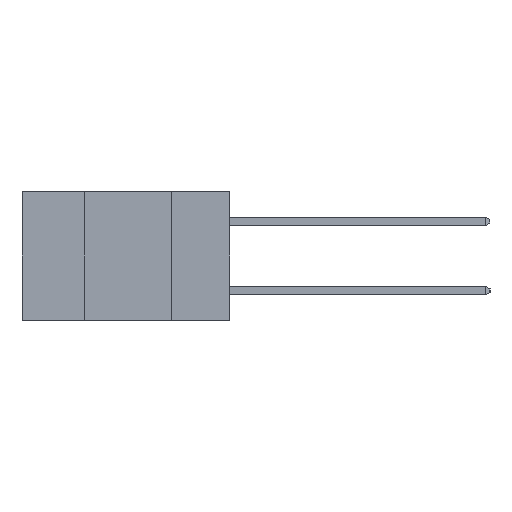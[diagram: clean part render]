
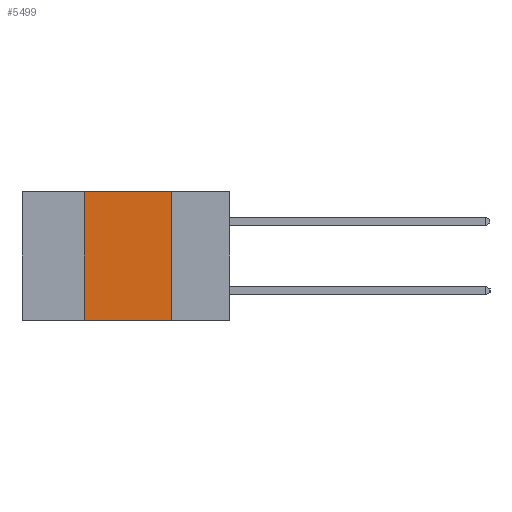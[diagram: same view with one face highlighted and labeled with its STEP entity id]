
A CAD part, left-side view. The second image highlights one B-rep face of the part: STEP entity #5499.
In plain terms, the highlighted planar face has unit normal (-1, 0, 0).
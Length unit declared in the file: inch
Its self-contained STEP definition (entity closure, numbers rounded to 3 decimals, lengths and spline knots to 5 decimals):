
#101 = VERTEX_POINT ( 'NONE', #11508 ) ;
#403 = DIRECTION ( 'NONE',  ( 0., 0., -1. ) ) ;
#486 = DIRECTION ( 'NONE',  ( 1., 0., 0. ) ) ;
#508 = PLANE ( 'NONE',  #15251 ) ;
#570 = CARTESIAN_POINT ( 'NONE',  ( 0., 0.6, 0. ) ) ;
#676 = VECTOR ( 'NONE', #7480, 39.37008 ) ;
#888 = FACE_OUTER_BOUND ( 'NONE', #13415, .T. ) ;
#1629 = VECTOR ( 'NONE', #9463, 39.37008 ) ;
#2603 = ORIENTED_EDGE ( 'NONE', *, *, #8192, .T. ) ;
#3342 = VERTEX_POINT ( 'NONE', #12175 ) ;
#4489 = ORIENTED_EDGE ( 'NONE', *, *, #6326, .F. ) ;
#4761 = LINE ( 'NONE', #9561, #1629 ) ;
#5140 = EDGE_CURVE ( 'NONE', #3342, #6577, #12088, .T. ) ;
#5459 = VECTOR ( 'NONE', #12535, 39.37008 ) ;
#5499 = ADVANCED_FACE ( 'NONE', ( #888 ), #508, .F. ) ;
#6326 = EDGE_CURVE ( 'NONE', #9936, #3342, #4761, .T. ) ;
#6577 = VERTEX_POINT ( 'NONE', #15065 ) ;
#6643 = EDGE_CURVE ( 'NONE', #6577, #101, #12986, .T. ) ;
#7480 = DIRECTION ( 'NONE',  ( 0., 0., -1. ) ) ;
#7483 = CARTESIAN_POINT ( 'NONE',  ( 0., 0.17, -0.37 ) ) ;
#7535 = LINE ( 'NONE', #12810, #5459 ) ;
#7576 = DIRECTION ( 'NONE',  ( 0., -1., 0. ) ) ;
#7886 = ORIENTED_EDGE ( 'NONE', *, *, #6643, .F. ) ;
#7955 = CARTESIAN_POINT ( 'NONE',  ( 0., 0.6, 0. ) ) ;
#8192 = EDGE_CURVE ( 'NONE', #9936, #101, #7535, .T. ) ;
#8976 = VECTOR ( 'NONE', #7576, 39.37008 ) ;
#9418 = ORIENTED_EDGE ( 'NONE', *, *, #5140, .F. ) ;
#9463 = DIRECTION ( 'NONE',  ( 0., 0., 1. ) ) ;
#9561 = CARTESIAN_POINT ( 'NONE',  ( 0., 0.42, -0.37 ) ) ;
#9936 = VERTEX_POINT ( 'NONE', #10465 ) ;
#10465 = CARTESIAN_POINT ( 'NONE',  ( 0., 0.42, -0.37 ) ) ;
#11508 = CARTESIAN_POINT ( 'NONE',  ( 0., 0.17, -0.37 ) ) ;
#12088 = LINE ( 'NONE', #7955, #8976 ) ;
#12175 = CARTESIAN_POINT ( 'NONE',  ( 0., 0.42, 0. ) ) ;
#12535 = DIRECTION ( 'NONE',  ( 0., -1., 0. ) ) ;
#12810 = CARTESIAN_POINT ( 'NONE',  ( 0., 0.6, -0.37 ) ) ;
#12986 = LINE ( 'NONE', #7483, #676 ) ;
#13415 = EDGE_LOOP ( 'NONE', ( #7886, #9418, #4489, #2603 ) ) ;
#15065 = CARTESIAN_POINT ( 'NONE',  ( 0., 0.17, 0. ) ) ;
#15251 = AXIS2_PLACEMENT_3D ( 'NONE', #570, #486, #403 ) ;
